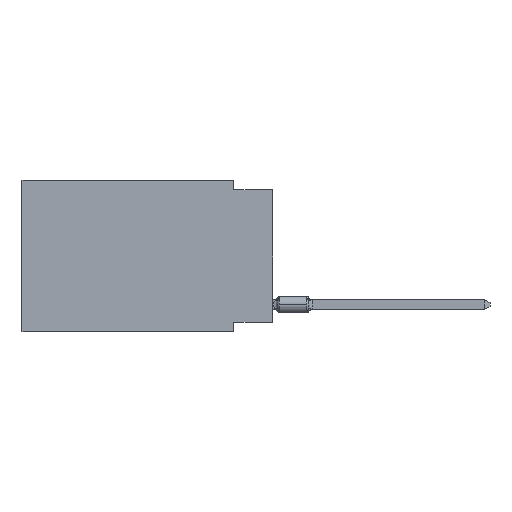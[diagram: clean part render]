
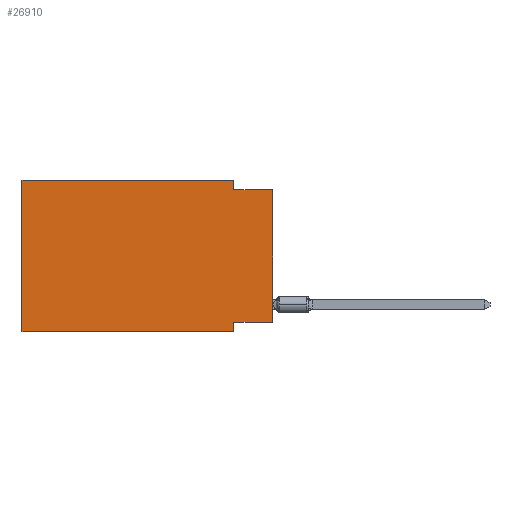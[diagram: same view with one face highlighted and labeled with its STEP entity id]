
A CAD part, left-side view. The second image highlights one B-rep face of the part: STEP entity #26910.
In plain terms, the highlighted planar face has unit normal (-1, 0, 0).
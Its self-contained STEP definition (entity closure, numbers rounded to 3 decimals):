
#725 = VECTOR ( 'NONE', #29183, 1000. ) ;
#833 = CARTESIAN_POINT ( 'NONE',  ( 0., 2.54, 0. ) ) ;
#1579 = EDGE_CURVE ( 'NONE', #10742, #12684, #13959, .T. ) ;
#2399 = LINE ( 'NONE', #15022, #29493 ) ;
#3161 = EDGE_CURVE ( 'NONE', #8324, #12684, #23859, .T. ) ;
#3289 = ORIENTED_EDGE ( 'NONE', *, *, #25966, .F. ) ;
#3696 = CARTESIAN_POINT ( 'NONE',  ( 0., 0., -0.635 ) ) ;
#6607 = VERTEX_POINT ( 'NONE', #22338 ) ;
#6738 = CARTESIAN_POINT ( 'NONE',  ( 0., 0., 0. ) ) ;
#6984 = AXIS2_PLACEMENT_3D ( 'NONE', #29570, #20038, #14878 ) ;
#7738 = ORIENTED_EDGE ( 'NONE', *, *, #3161, .F. ) ;
#8324 = VERTEX_POINT ( 'NONE', #23947 ) ;
#8992 = CARTESIAN_POINT ( 'NONE',  ( 0., 16.383, -9.906 ) ) ;
#9515 = VECTOR ( 'NONE', #30697, 1000. ) ;
#9646 = CARTESIAN_POINT ( 'NONE',  ( 0., 2.54, 0. ) ) ;
#9686 = DIRECTION ( 'NONE',  ( 0., 0., 1. ) ) ;
#9744 = EDGE_CURVE ( 'NONE', #20972, #17985, #11497, .T. ) ;
#10742 = VERTEX_POINT ( 'NONE', #8992 ) ;
#11497 = LINE ( 'NONE', #28939, #17690 ) ;
#11896 = LINE ( 'NONE', #6738, #725 ) ;
#12010 = DIRECTION ( 'NONE',  ( 0., -1., 0. ) ) ;
#12194 = VECTOR ( 'NONE', #12010, 1000. ) ;
#12684 = VERTEX_POINT ( 'NONE', #24442 ) ;
#13959 = LINE ( 'NONE', #23820, #12194 ) ;
#14567 = ORIENTED_EDGE ( 'NONE', *, *, #14635, .F. ) ;
#14635 = EDGE_CURVE ( 'NONE', #17985, #18578, #26621, .T. ) ;
#14717 = PLANE ( 'NONE',  #6984 ) ;
#14797 = ORIENTED_EDGE ( 'NONE', *, *, #24378, .T. ) ;
#14878 = DIRECTION ( 'NONE',  ( 0., 0., -1. ) ) ;
#15022 = CARTESIAN_POINT ( 'NONE',  ( 0., 0., -9.271 ) ) ;
#15692 = ORIENTED_EDGE ( 'NONE', *, *, #1579, .T. ) ;
#15882 = VECTOR ( 'NONE', #31292, 1000. ) ;
#16136 = CARTESIAN_POINT ( 'NONE',  ( 0., 0., -0.635 ) ) ;
#17690 = VECTOR ( 'NONE', #31213, 1000. ) ;
#17866 = ORIENTED_EDGE ( 'NONE', *, *, #30783, .F. ) ;
#17985 = VERTEX_POINT ( 'NONE', #833 ) ;
#18578 = VERTEX_POINT ( 'NONE', #30049 ) ;
#18709 = LINE ( 'NONE', #16136, #9515 ) ;
#19688 = DIRECTION ( 'NONE',  ( 0., 1., 0. ) ) ;
#19699 = LINE ( 'NONE', #21653, #29610 ) ;
#20038 = DIRECTION ( 'NONE',  ( 1., 0., 0. ) ) ;
#20734 = EDGE_CURVE ( 'NONE', #6607, #8324, #2399, .T. ) ;
#20972 = VERTEX_POINT ( 'NONE', #28398 ) ;
#21441 = CARTESIAN_POINT ( 'NONE',  ( 0., 2.54, -9.906 ) ) ;
#21653 = CARTESIAN_POINT ( 'NONE',  ( 0., 16.383, 0. ) ) ;
#22338 = CARTESIAN_POINT ( 'NONE',  ( 0., 0., -9.271 ) ) ;
#22498 = ORIENTED_EDGE ( 'NONE', *, *, #9744, .F. ) ;
#22547 = EDGE_LOOP ( 'NONE', ( #14797, #3289, #14567, #22498, #17866, #15692, #7738, #28478 ) ) ;
#22591 = VECTOR ( 'NONE', #24041, 1000. ) ;
#23820 = CARTESIAN_POINT ( 'NONE',  ( 0., 16.383, -9.906 ) ) ;
#23859 = LINE ( 'NONE', #21441, #15882 ) ;
#23947 = CARTESIAN_POINT ( 'NONE',  ( 0., 2.54, -9.271 ) ) ;
#24041 = DIRECTION ( 'NONE',  ( 0., 0., -1. ) ) ;
#24378 = EDGE_CURVE ( 'NONE', #6607, #24925, #11896, .T. ) ;
#24442 = CARTESIAN_POINT ( 'NONE',  ( 0., 2.54, -9.906 ) ) ;
#24925 = VERTEX_POINT ( 'NONE', #3696 ) ;
#25966 = EDGE_CURVE ( 'NONE', #18578, #24925, #18709, .T. ) ;
#26621 = LINE ( 'NONE', #9646, #22591 ) ;
#26910 = ADVANCED_FACE ( 'NONE', ( #26981 ), #14717, .F. ) ;
#26981 = FACE_OUTER_BOUND ( 'NONE', #22547, .T. ) ;
#28398 = CARTESIAN_POINT ( 'NONE',  ( 0., 16.383, 0. ) ) ;
#28478 = ORIENTED_EDGE ( 'NONE', *, *, #20734, .F. ) ;
#28939 = CARTESIAN_POINT ( 'NONE',  ( 0., 16.383, 0. ) ) ;
#29183 = DIRECTION ( 'NONE',  ( 0., 0., 1. ) ) ;
#29493 = VECTOR ( 'NONE', #19688, 1000. ) ;
#29570 = CARTESIAN_POINT ( 'NONE',  ( 0., 16.383, 0. ) ) ;
#29610 = VECTOR ( 'NONE', #9686, 1000. ) ;
#30049 = CARTESIAN_POINT ( 'NONE',  ( 0., 2.54, -0.635 ) ) ;
#30697 = DIRECTION ( 'NONE',  ( 0., -1., 0. ) ) ;
#30783 = EDGE_CURVE ( 'NONE', #10742, #20972, #19699, .T. ) ;
#31213 = DIRECTION ( 'NONE',  ( 0., -1., 0. ) ) ;
#31292 = DIRECTION ( 'NONE',  ( 0., 0., -1. ) ) ;
